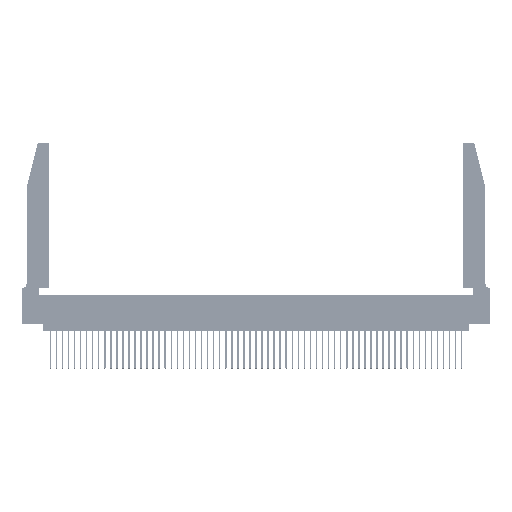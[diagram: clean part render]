
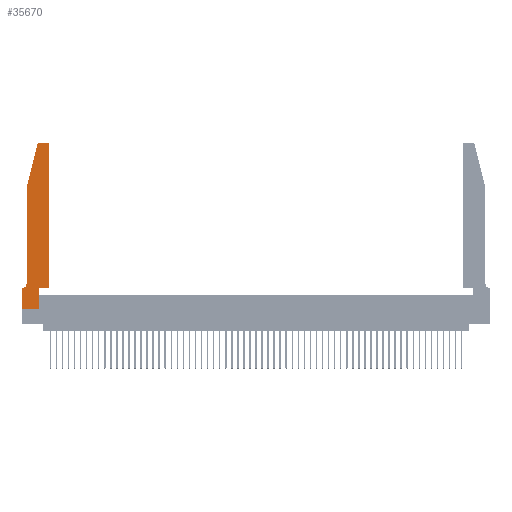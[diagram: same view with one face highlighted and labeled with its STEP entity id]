
A CAD part, top view. The second image highlights one B-rep face of the part: STEP entity #35670.
In plain terms, the highlighted planar face has unit normal (0, 0, 1).
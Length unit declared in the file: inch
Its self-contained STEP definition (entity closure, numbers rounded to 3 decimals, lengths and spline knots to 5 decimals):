
#395 = DIRECTION ( 'NONE',  ( 1., 0., 0. ) ) ;
#580 = CARTESIAN_POINT ( 'NONE',  ( 0.284, 2.72, 0.37 ) ) ;
#673 = VECTOR ( 'NONE', #44623, 39.37008 ) ;
#1403 = DIRECTION ( 'NONE',  ( 0., 1., 0. ) ) ;
#1639 = AXIS2_PLACEMENT_3D ( 'NONE', #53690, #19191, #44866 ) ;
#2137 = VERTEX_POINT ( 'NONE', #25815 ) ;
#2166 = EDGE_CURVE ( 'NONE', #18997, #15919, #14688, .T. ) ;
#3939 = EDGE_CURVE ( 'NONE', #16552, #18997, #54440, .T. ) ;
#4130 = DIRECTION ( 'NONE',  ( 0., 0., 1. ) ) ;
#5098 = DIRECTION ( 'NONE',  ( 0., 0., 1. ) ) ;
#5551 = CARTESIAN_POINT ( 'NONE',  ( 0., 0., 0.37 ) ) ;
#5576 = ORIENTED_EDGE ( 'NONE', *, *, #37244, .T. ) ;
#5691 = ORIENTED_EDGE ( 'NONE', *, *, #2166, .T. ) ;
#6390 = ORIENTED_EDGE ( 'NONE', *, *, #45953, .T. ) ;
#6463 = LINE ( 'NONE', #47795, #29186 ) ;
#8977 = CARTESIAN_POINT ( 'NONE',  ( 0.2865, 0.35, 0.37 ) ) ;
#9125 = VERTEX_POINT ( 'NONE', #29632 ) ;
#9365 = DIRECTION ( 'NONE',  ( 1., 0., 0. ) ) ;
#9653 = ORIENTED_EDGE ( 'NONE', *, *, #36197, .T. ) ;
#10576 = CIRCLE ( 'NONE', #1639, 0.03 ) ;
#12246 = LINE ( 'NONE', #28770, #41777 ) ;
#13229 = EDGE_CURVE ( 'NONE', #51675, #47578, #32790, .T. ) ;
#13469 = VECTOR ( 'NONE', #31522, 39.37008 ) ;
#14688 = LINE ( 'NONE', #48100, #26098 ) ;
#15032 = VERTEX_POINT ( 'NONE', #52158 ) ;
#15467 = EDGE_CURVE ( 'NONE', #31375, #15032, #39288, .T. ) ;
#15919 = VERTEX_POINT ( 'NONE', #41020 ) ;
#16552 = VERTEX_POINT ( 'NONE', #24005 ) ;
#18997 = VERTEX_POINT ( 'NONE', #33433 ) ;
#19187 = EDGE_CURVE ( 'NONE', #2137, #51675, #24855, .T. ) ;
#19191 = DIRECTION ( 'NONE',  ( 0., 0., 1. ) ) ;
#19307 = CARTESIAN_POINT ( 'NONE',  ( 0.0755, 0.35, 0.37 ) ) ;
#19436 = ORIENTED_EDGE ( 'NONE', *, *, #47162, .T. ) ;
#19495 = VECTOR ( 'NONE', #41792, 39.37008 ) ;
#21004 = CARTESIAN_POINT ( 'NONE',  ( 0.0055, 0.42, 0.37 ) ) ;
#22639 = CARTESIAN_POINT ( 'NONE',  ( 0., 0.35, 0.37 ) ) ;
#23832 = VECTOR ( 'NONE', #29238, 39.37008 ) ;
#24005 = CARTESIAN_POINT ( 'NONE',  ( 0.284, 2.75, 0.37 ) ) ;
#24855 = LINE ( 'NONE', #19307, #13469 ) ;
#24924 = CARTESIAN_POINT ( 'NONE',  ( 0.4505, 0.35, 0.37 ) ) ;
#25153 = DIRECTION ( 'NONE',  ( 0., -1., 0. ) ) ;
#25815 = CARTESIAN_POINT ( 'NONE',  ( 0.0055, 0.35, 0.37 ) ) ;
#26098 = VECTOR ( 'NONE', #29139, 39.37008 ) ;
#26160 = ORIENTED_EDGE ( 'NONE', *, *, #27775, .T. ) ;
#26250 = LINE ( 'NONE', #46060, #19495 ) ;
#26570 = VERTEX_POINT ( 'NONE', #42541 ) ;
#27590 = VERTEX_POINT ( 'NONE', #37346 ) ;
#27775 = EDGE_CURVE ( 'NONE', #9125, #2137, #40205, .T. ) ;
#28749 = EDGE_CURVE ( 'NONE', #26570, #27590, #10576, .T. ) ;
#28770 = CARTESIAN_POINT ( 'NONE',  ( 0.2865, 0.35, 0.37 ) ) ;
#29139 = DIRECTION ( 'NONE',  ( -0.239, -0.971, 0. ) ) ;
#29186 = VECTOR ( 'NONE', #1403, 39.37008 ) ;
#29238 = DIRECTION ( 'NONE',  ( 1., 0., 0. ) ) ;
#29533 = VECTOR ( 'NONE', #25153, 39.37008 ) ;
#29632 = CARTESIAN_POINT ( 'NONE',  ( 0.0755, 0.42, 0.37 ) ) ;
#30416 = ORIENTED_EDGE ( 'NONE', *, *, #15467, .T. ) ;
#31355 = EDGE_LOOP ( 'NONE', ( #19436, #53217, #5691, #43682, #26160, #54244, #42562, #5576, #9653, #30416, #6390, #33554 ) ) ;
#31375 = VERTEX_POINT ( 'NONE', #8977 ) ;
#31522 = DIRECTION ( 'NONE',  ( -1., 0., 0. ) ) ;
#31677 = AXIS2_PLACEMENT_3D ( 'NONE', #21004, #33766, #42402 ) ;
#32790 = LINE ( 'NONE', #5551, #673 ) ;
#33433 = CARTESIAN_POINT ( 'NONE',  ( 0.25487, 2.72718, 0.37 ) ) ;
#33467 = FACE_OUTER_BOUND ( 'NONE', #31355, .T. ) ;
#33554 = ORIENTED_EDGE ( 'NONE', *, *, #28749, .T. ) ;
#33766 = DIRECTION ( 'NONE',  ( 0., 0., -1. ) ) ;
#34920 = EDGE_CURVE ( 'NONE', #15919, #9125, #42301, .T. ) ;
#35384 = CARTESIAN_POINT ( 'NONE',  ( 0., 0.35, 0.37 ) ) ;
#35670 = ADVANCED_FACE ( 'NONE', ( #33467 ), #48314, .T. ) ;
#36197 = EDGE_CURVE ( 'NONE', #39881, #31375, #12246, .T. ) ;
#37244 = EDGE_CURVE ( 'NONE', #47578, #39881, #26250, .T. ) ;
#37346 = CARTESIAN_POINT ( 'NONE',  ( 0.4205, 2.75, 0.37 ) ) ;
#37701 = CARTESIAN_POINT ( 'NONE',  ( 0.0755, 2., 0.37 ) ) ;
#37723 = AXIS2_PLACEMENT_3D ( 'NONE', #580, #4130, #395 ) ;
#39288 = LINE ( 'NONE', #24924, #23832 ) ;
#39881 = VERTEX_POINT ( 'NONE', #42043 ) ;
#40205 = CIRCLE ( 'NONE', #31677, 0.07 ) ;
#41020 = CARTESIAN_POINT ( 'NONE',  ( 0.0755, 2., 0.37 ) ) ;
#41777 = VECTOR ( 'NONE', #41907, 39.37008 ) ;
#41792 = DIRECTION ( 'NONE',  ( 1., 0., 0. ) ) ;
#41907 = DIRECTION ( 'NONE',  ( 0., 1., 0. ) ) ;
#42043 = CARTESIAN_POINT ( 'NONE',  ( 0.2865, 0., 0.37 ) ) ;
#42301 = LINE ( 'NONE', #37701, #29533 ) ;
#42402 = DIRECTION ( 'NONE',  ( -1., 0., 0. ) ) ;
#42541 = CARTESIAN_POINT ( 'NONE',  ( 0.4505, 2.72, 0.37 ) ) ;
#42562 = ORIENTED_EDGE ( 'NONE', *, *, #13229, .T. ) ;
#43154 = CARTESIAN_POINT ( 'NONE',  ( 0.2605, 2.75, 0.37 ) ) ;
#43682 = ORIENTED_EDGE ( 'NONE', *, *, #34920, .T. ) ;
#44623 = DIRECTION ( 'NONE',  ( 0., -1., 0. ) ) ;
#44866 = DIRECTION ( 'NONE',  ( 1., 0., 0. ) ) ;
#45103 = VECTOR ( 'NONE', #47426, 39.37008 ) ;
#45438 = AXIS2_PLACEMENT_3D ( 'NONE', #35384, #5098, #9365 ) ;
#45695 = CARTESIAN_POINT ( 'NONE',  ( 0., 0., 0.37 ) ) ;
#45953 = EDGE_CURVE ( 'NONE', #15032, #26570, #6463, .T. ) ;
#46060 = CARTESIAN_POINT ( 'NONE',  ( 0., 0., 0.37 ) ) ;
#47162 = EDGE_CURVE ( 'NONE', #27590, #16552, #49154, .T. ) ;
#47426 = DIRECTION ( 'NONE',  ( -1., 0., 0. ) ) ;
#47578 = VERTEX_POINT ( 'NONE', #45695 ) ;
#47795 = CARTESIAN_POINT ( 'NONE',  ( 0.4505, 0.35, 0.37 ) ) ;
#48100 = CARTESIAN_POINT ( 'NONE',  ( 0.0755, 2., 0.37 ) ) ;
#48314 = PLANE ( 'NONE',  #45438 ) ;
#49154 = LINE ( 'NONE', #43154, #45103 ) ;
#51675 = VERTEX_POINT ( 'NONE', #22639 ) ;
#52158 = CARTESIAN_POINT ( 'NONE',  ( 0.4505, 0.35, 0.37 ) ) ;
#53217 = ORIENTED_EDGE ( 'NONE', *, *, #3939, .T. ) ;
#53690 = CARTESIAN_POINT ( 'NONE',  ( 0.4205, 2.72, 0.37 ) ) ;
#54244 = ORIENTED_EDGE ( 'NONE', *, *, #19187, .T. ) ;
#54440 = CIRCLE ( 'NONE', #37723, 0.03 ) ;
